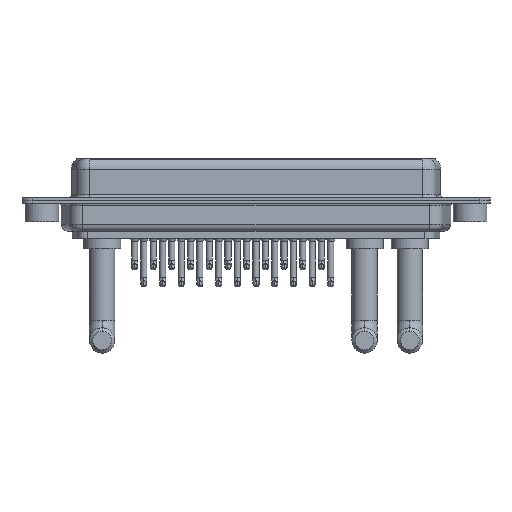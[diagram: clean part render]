
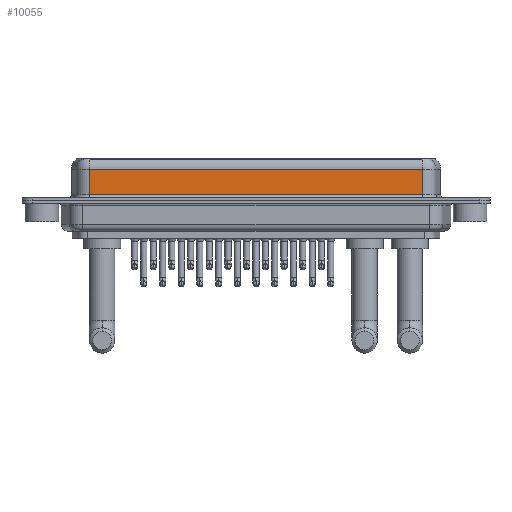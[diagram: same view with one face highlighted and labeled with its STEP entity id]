
A CAD part, front view. The second image highlights one B-rep face of the part: STEP entity #10055.
In plain terms, the highlighted planar face has unit normal (0, -1, 0).
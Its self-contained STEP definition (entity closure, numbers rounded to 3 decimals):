
#914 = EDGE_CURVE ( 'NONE', #22484, #10404, #3380, .T. ) ;
#1270 = VERTEX_POINT ( 'NONE', #22870 ) ;
#3087 = DIRECTION ( 'NONE',  ( 0., 0., 1. ) ) ;
#3208 = CARTESIAN_POINT ( 'NONE',  ( 56.462, -3.95, 6.4 ) ) ;
#3324 = CARTESIAN_POINT ( 'NONE',  ( 56.462, -3.95, 6.4 ) ) ;
#3380 = LINE ( 'NONE', #23598, #3544 ) ;
#3544 = VECTOR ( 'NONE', #14564, 1000. ) ;
#3761 = CARTESIAN_POINT ( 'NONE',  ( 56.462, -3.95, 4.65 ) ) ;
#4032 = EDGE_CURVE ( 'NONE', #1270, #5187, #20789, .T. ) ;
#4789 = EDGE_CURVE ( 'NONE', #10404, #1270, #15944, .T. ) ;
#5023 = DIRECTION ( 'NONE',  ( 0., 0., -1. ) ) ;
#5187 = VERTEX_POINT ( 'NONE', #20751 ) ;
#5372 = VECTOR ( 'NONE', #7689, 1000. ) ;
#6320 = ORIENTED_EDGE ( 'NONE', *, *, #10022, .F. ) ;
#6341 = VECTOR ( 'NONE', #5023, 1000. ) ;
#7689 = DIRECTION ( 'NONE',  ( 1., 0., 0. ) ) ;
#9137 = ORIENTED_EDGE ( 'NONE', *, *, #4789, .T. ) ;
#10022 = EDGE_CURVE ( 'NONE', #22484, #5187, #14143, .T. ) ;
#10055 = ADVANCED_FACE ( 'NONE', ( #14261 ), #19571, .F. ) ;
#10404 = VERTEX_POINT ( 'NONE', #19417 ) ;
#12036 = ORIENTED_EDGE ( 'NONE', *, *, #4032, .T. ) ;
#12841 = AXIS2_PLACEMENT_3D ( 'NONE', #3324, #14509, #3087 ) ;
#14143 = LINE ( 'NONE', #3208, #6341 ) ;
#14261 = FACE_OUTER_BOUND ( 'NONE', #22352, .T. ) ;
#14509 = DIRECTION ( 'NONE',  ( 0., 1., 0. ) ) ;
#14564 = DIRECTION ( 'NONE',  ( -1., 0., 0. ) ) ;
#15944 = LINE ( 'NONE', #21388, #16147 ) ;
#16147 = VECTOR ( 'NONE', #17759, 1000. ) ;
#17168 = CARTESIAN_POINT ( 'NONE',  ( 56.462, -3.95, 0.9 ) ) ;
#17759 = DIRECTION ( 'NONE',  ( 0., 0., -1. ) ) ;
#18090 = ORIENTED_EDGE ( 'NONE', *, *, #914, .T. ) ;
#19417 = CARTESIAN_POINT ( 'NONE',  ( 7.038, -3.95, 4.65 ) ) ;
#19571 = PLANE ( 'NONE',  #12841 ) ;
#20751 = CARTESIAN_POINT ( 'NONE',  ( 56.462, -3.95, 0.9 ) ) ;
#20789 = LINE ( 'NONE', #17168, #5372 ) ;
#21388 = CARTESIAN_POINT ( 'NONE',  ( 7.038, -3.95, 6.4 ) ) ;
#22352 = EDGE_LOOP ( 'NONE', ( #6320, #18090, #9137, #12036 ) ) ;
#22484 = VERTEX_POINT ( 'NONE', #3761 ) ;
#22870 = CARTESIAN_POINT ( 'NONE',  ( 7.038, -3.95, 0.9 ) ) ;
#23598 = CARTESIAN_POINT ( 'NONE',  ( 56.462, -3.95, 4.65 ) ) ;
